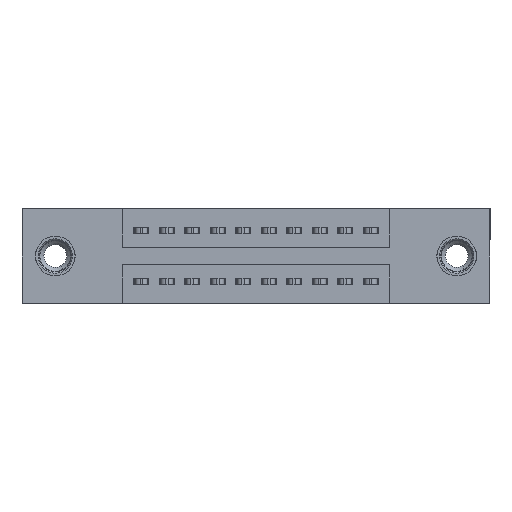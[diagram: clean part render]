
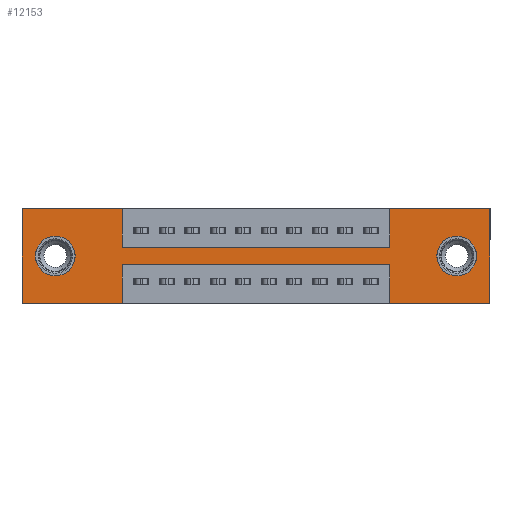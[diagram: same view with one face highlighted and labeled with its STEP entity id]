
A CAD part, front view. The second image highlights one B-rep face of the part: STEP entity #12153.
In plain terms, the highlighted planar face has unit normal (0, -1, 0).
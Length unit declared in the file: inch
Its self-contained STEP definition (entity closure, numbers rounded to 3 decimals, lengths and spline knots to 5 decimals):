
#31 = EDGE_CURVE ( 'NONE', #2342, #12532, #11662, .T. ) ;
#251 = EDGE_CURVE ( 'NONE', #15016, #5194, #14957, .T. ) ;
#276 = EDGE_CURVE ( 'NONE', #3164, #9824, #1119, .T. ) ;
#280 = EDGE_LOOP ( 'NONE', ( #573, #8255 ) ) ;
#285 = VECTOR ( 'NONE', #16193, 39.37008 ) ;
#544 = ORIENTED_EDGE ( 'NONE', *, *, #11384, .T. ) ;
#573 = ORIENTED_EDGE ( 'NONE', *, *, #6864, .T. ) ;
#777 = ORIENTED_EDGE ( 'NONE', *, *, #975, .F. ) ;
#886 = FACE_OUTER_BOUND ( 'NONE', #4533, .T. ) ;
#938 = VECTOR ( 'NONE', #4726, 39.37008 ) ;
#975 = EDGE_CURVE ( 'NONE', #16140, #8398, #4770, .T. ) ;
#992 = ORIENTED_EDGE ( 'NONE', *, *, #7786, .F. ) ;
#1119 = LINE ( 'NONE', #2322, #3166 ) ;
#1150 = CARTESIAN_POINT ( 'NONE',  ( 0., 0., 0. ) ) ;
#1235 = CARTESIAN_POINT ( 'NONE',  ( 1.4425, 0., 0. ) ) ;
#1354 = CIRCLE ( 'NONE', #9158, 0.078 ) ;
#1356 = DIRECTION ( 'NONE',  ( 0., 1., 0. ) ) ;
#1519 = EDGE_CURVE ( 'NONE', #4421, #15016, #8809, .T. ) ;
#1621 = ORIENTED_EDGE ( 'NONE', *, *, #251, .F. ) ;
#1656 = DIRECTION ( 'NONE',  ( 0., 1., 0. ) ) ;
#1992 = DIRECTION ( 'NONE',  ( 0., 0., -1. ) ) ;
#2018 = DIRECTION ( 'NONE',  ( 0., 0., 1. ) ) ;
#2179 = VECTOR ( 'NONE', #15319, 39.37008 ) ;
#2322 = CARTESIAN_POINT ( 'NONE',  ( 0.3925, 0., -0.22 ) ) ;
#2342 = VERTEX_POINT ( 'NONE', #11718 ) ;
#2347 = CARTESIAN_POINT ( 'NONE',  ( 0.3925, 0., 0. ) ) ;
#2508 = VECTOR ( 'NONE', #5068, 39.37008 ) ;
#2899 = VECTOR ( 'NONE', #3785, 39.37008 ) ;
#3164 = VERTEX_POINT ( 'NONE', #13243 ) ;
#3166 = VECTOR ( 'NONE', #9085, 39.37008 ) ;
#3217 = DIRECTION ( 'NONE',  ( 0., 1., 0. ) ) ;
#3661 = AXIS2_PLACEMENT_3D ( 'NONE', #6236, #16677, #3714 ) ;
#3714 = DIRECTION ( 'NONE',  ( 0., 0., -1. ) ) ;
#3765 = CARTESIAN_POINT ( 'NONE',  ( 0.3925, 0., -0.37 ) ) ;
#3785 = DIRECTION ( 'NONE',  ( 1., 0., 0. ) ) ;
#3853 = DIRECTION ( 'NONE',  ( 0., 0., 1. ) ) ;
#4122 = ORIENTED_EDGE ( 'NONE', *, *, #12115, .F. ) ;
#4421 = VERTEX_POINT ( 'NONE', #4843 ) ;
#4533 = EDGE_LOOP ( 'NONE', ( #4122, #4898, #6753, #11681, #7192, #992, #777, #6860, #8743, #12164, #1621, #9270 ) ) ;
#4624 = CARTESIAN_POINT ( 'NONE',  ( 1.4425, 0., -0.37 ) ) ;
#4695 = CARTESIAN_POINT ( 'NONE',  ( 0., 0., -0.37 ) ) ;
#4726 = DIRECTION ( 'NONE',  ( 0., 0., -1. ) ) ;
#4770 = LINE ( 'NONE', #13941, #12863 ) ;
#4843 = CARTESIAN_POINT ( 'NONE',  ( 0.3925, 0., -0.37 ) ) ;
#4898 = ORIENTED_EDGE ( 'NONE', *, *, #276, .F. ) ;
#5068 = DIRECTION ( 'NONE',  ( 0., 0., -1. ) ) ;
#5194 = VERTEX_POINT ( 'NONE', #5394 ) ;
#5236 = VERTEX_POINT ( 'NONE', #13610 ) ;
#5294 = DIRECTION ( 'NONE',  ( -1., 0., 0. ) ) ;
#5394 = CARTESIAN_POINT ( 'NONE',  ( 0., 0., 0. ) ) ;
#5460 = ORIENTED_EDGE ( 'NONE', *, *, #10456, .T. ) ;
#5500 = AXIS2_PLACEMENT_3D ( 'NONE', #8388, #3217, #1992 ) ;
#5793 = VERTEX_POINT ( 'NONE', #4624 ) ;
#5794 = LINE ( 'NONE', #10860, #5997 ) ;
#5814 = VERTEX_POINT ( 'NONE', #12477 ) ;
#5997 = VECTOR ( 'NONE', #16122, 39.37008 ) ;
#6117 = CARTESIAN_POINT ( 'NONE',  ( 0., 0., 0. ) ) ;
#6236 = CARTESIAN_POINT ( 'NONE',  ( 0., 0., -0.37 ) ) ;
#6437 = EDGE_CURVE ( 'NONE', #10852, #16140, #12509, .T. ) ;
#6570 = CARTESIAN_POINT ( 'NONE',  ( 1.4425, 0., -0.15 ) ) ;
#6747 = DIRECTION ( 'NONE',  ( 0., 0., -1. ) ) ;
#6753 = ORIENTED_EDGE ( 'NONE', *, *, #14354, .F. ) ;
#6860 = ORIENTED_EDGE ( 'NONE', *, *, #6437, .F. ) ;
#6864 = EDGE_CURVE ( 'NONE', #12532, #2342, #1354, .T. ) ;
#7026 = EDGE_CURVE ( 'NONE', #11265, #5814, #11696, .T. ) ;
#7164 = CARTESIAN_POINT ( 'NONE',  ( 1.4425, 0., -0.37 ) ) ;
#7192 = ORIENTED_EDGE ( 'NONE', *, *, #7026, .F. ) ;
#7195 = DIRECTION ( 'NONE',  ( 0., 0., 1. ) ) ;
#7236 = DIRECTION ( 'NONE',  ( 0., 0., 1. ) ) ;
#7390 = CARTESIAN_POINT ( 'NONE',  ( 0.3925, 0., 0. ) ) ;
#7434 = VECTOR ( 'NONE', #16606, 39.37008 ) ;
#7529 = EDGE_CURVE ( 'NONE', #9348, #10852, #10088, .T. ) ;
#7729 = CIRCLE ( 'NONE', #15963, 0.078 ) ;
#7786 = EDGE_CURVE ( 'NONE', #8398, #11265, #5794, .T. ) ;
#8200 = FACE_BOUND ( 'NONE', #13391, .T. ) ;
#8255 = ORIENTED_EDGE ( 'NONE', *, *, #31, .T. ) ;
#8388 = CARTESIAN_POINT ( 'NONE',  ( 1.705, 0., -0.185 ) ) ;
#8398 = VERTEX_POINT ( 'NONE', #1235 ) ;
#8523 = CARTESIAN_POINT ( 'NONE',  ( 1.705, 0., -0.263 ) ) ;
#8743 = ORIENTED_EDGE ( 'NONE', *, *, #7529, .F. ) ;
#8809 = LINE ( 'NONE', #12432, #285 ) ;
#8859 = EDGE_CURVE ( 'NONE', #5814, #5793, #10440, .T. ) ;
#9085 = DIRECTION ( 'NONE',  ( -1., 0., 0. ) ) ;
#9158 = AXIS2_PLACEMENT_3D ( 'NONE', #16408, #9750, #7195 ) ;
#9225 = VECTOR ( 'NONE', #5294, 39.37008 ) ;
#9270 = ORIENTED_EDGE ( 'NONE', *, *, #1519, .F. ) ;
#9279 = CARTESIAN_POINT ( 'NONE',  ( 0.3925, 0., -0.22 ) ) ;
#9348 = VERTEX_POINT ( 'NONE', #2347 ) ;
#9446 = CARTESIAN_POINT ( 'NONE',  ( 0.13, 0., -0.185 ) ) ;
#9750 = DIRECTION ( 'NONE',  ( 0., 1., 0. ) ) ;
#9824 = VERTEX_POINT ( 'NONE', #9279 ) ;
#10088 = LINE ( 'NONE', #7390, #938 ) ;
#10350 = PLANE ( 'NONE',  #3661 ) ;
#10440 = LINE ( 'NONE', #14344, #9225 ) ;
#10449 = CARTESIAN_POINT ( 'NONE',  ( 1.705, 0., -0.185 ) ) ;
#10456 = EDGE_CURVE ( 'NONE', #14316, #5236, #7729, .T. ) ;
#10603 = CARTESIAN_POINT ( 'NONE',  ( 1.835, 0., 0. ) ) ;
#10852 = VERTEX_POINT ( 'NONE', #15169 ) ;
#10860 = CARTESIAN_POINT ( 'NONE',  ( 0., 0., 0. ) ) ;
#11265 = VERTEX_POINT ( 'NONE', #10603 ) ;
#11355 = CIRCLE ( 'NONE', #5500, 0.078 ) ;
#11384 = EDGE_CURVE ( 'NONE', #5236, #14316, #11355, .T. ) ;
#11662 = CIRCLE ( 'NONE', #16305, 0.078 ) ;
#11681 = ORIENTED_EDGE ( 'NONE', *, *, #8859, .F. ) ;
#11696 = LINE ( 'NONE', #11990, #11888 ) ;
#11718 = CARTESIAN_POINT ( 'NONE',  ( 0.13, 0., -0.263 ) ) ;
#11888 = VECTOR ( 'NONE', #6747, 39.37008 ) ;
#11990 = CARTESIAN_POINT ( 'NONE',  ( 1.835, 0., 0. ) ) ;
#12031 = LINE ( 'NONE', #3765, #2508 ) ;
#12115 = EDGE_CURVE ( 'NONE', #9824, #4421, #12031, .T. ) ;
#12153 = ADVANCED_FACE ( 'NONE', ( #8200, #15944, #886 ), #10350, .T. ) ;
#12164 = ORIENTED_EDGE ( 'NONE', *, *, #12505, .F. ) ;
#12432 = CARTESIAN_POINT ( 'NONE',  ( 0., 0., -0.37 ) ) ;
#12477 = CARTESIAN_POINT ( 'NONE',  ( 1.835, 0., -0.37 ) ) ;
#12505 = EDGE_CURVE ( 'NONE', #5194, #9348, #13255, .T. ) ;
#12509 = LINE ( 'NONE', #13923, #2179 ) ;
#12532 = VERTEX_POINT ( 'NONE', #14946 ) ;
#12863 = VECTOR ( 'NONE', #3853, 39.37008 ) ;
#13243 = CARTESIAN_POINT ( 'NONE',  ( 1.4425, 0., -0.22 ) ) ;
#13255 = LINE ( 'NONE', #1150, #2899 ) ;
#13391 = EDGE_LOOP ( 'NONE', ( #544, #5460 ) ) ;
#13410 = VECTOR ( 'NONE', #2018, 39.37008 ) ;
#13610 = CARTESIAN_POINT ( 'NONE',  ( 1.705, 0., -0.107 ) ) ;
#13923 = CARTESIAN_POINT ( 'NONE',  ( 0.3925, 0., -0.15 ) ) ;
#13941 = CARTESIAN_POINT ( 'NONE',  ( 1.4425, 0., 0. ) ) ;
#14316 = VERTEX_POINT ( 'NONE', #8523 ) ;
#14344 = CARTESIAN_POINT ( 'NONE',  ( 0., 0., -0.37 ) ) ;
#14354 = EDGE_CURVE ( 'NONE', #5793, #3164, #15481, .T. ) ;
#14946 = CARTESIAN_POINT ( 'NONE',  ( 0.13, 0., -0.107 ) ) ;
#14957 = LINE ( 'NONE', #6117, #7434 ) ;
#15016 = VERTEX_POINT ( 'NONE', #4695 ) ;
#15169 = CARTESIAN_POINT ( 'NONE',  ( 0.3925, 0., -0.15 ) ) ;
#15319 = DIRECTION ( 'NONE',  ( 1., 0., 0. ) ) ;
#15418 = DIRECTION ( 'NONE',  ( 0., 0., -1. ) ) ;
#15481 = LINE ( 'NONE', #7164, #13410 ) ;
#15944 = FACE_BOUND ( 'NONE', #280, .T. ) ;
#15963 = AXIS2_PLACEMENT_3D ( 'NONE', #10449, #1356, #15418 ) ;
#16122 = DIRECTION ( 'NONE',  ( 1., 0., 0. ) ) ;
#16140 = VERTEX_POINT ( 'NONE', #6570 ) ;
#16193 = DIRECTION ( 'NONE',  ( -1., 0., 0. ) ) ;
#16305 = AXIS2_PLACEMENT_3D ( 'NONE', #9446, #1656, #7236 ) ;
#16408 = CARTESIAN_POINT ( 'NONE',  ( 0.13, 0., -0.185 ) ) ;
#16606 = DIRECTION ( 'NONE',  ( 0., 0., 1. ) ) ;
#16677 = DIRECTION ( 'NONE',  ( 0., -1., 0. ) ) ;
